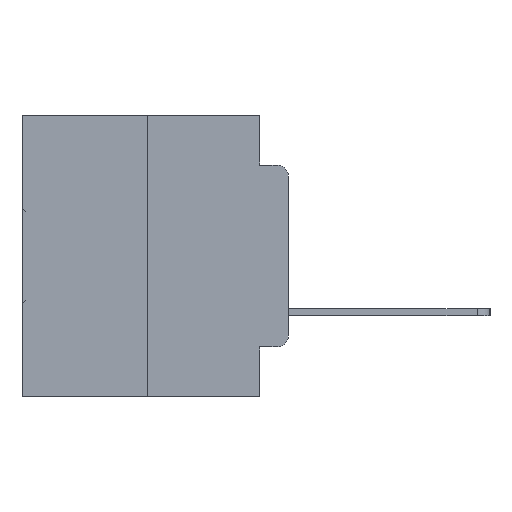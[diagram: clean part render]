
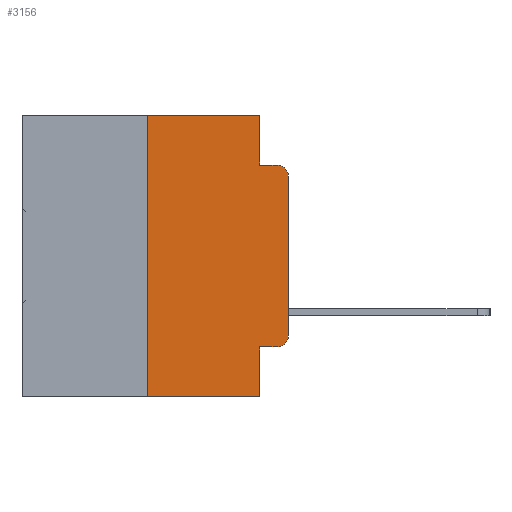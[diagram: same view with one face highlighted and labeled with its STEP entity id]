
A CAD part, left-side view. The second image highlights one B-rep face of the part: STEP entity #3156.
In plain terms, the highlighted planar face has unit normal (-1, 0, 0).
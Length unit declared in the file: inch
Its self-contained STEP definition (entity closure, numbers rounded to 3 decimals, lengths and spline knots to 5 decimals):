
#2211 = ORIENTED_EDGE ( 'NONE', *, *, #18443, .T. ) ;
#2408 = CARTESIAN_POINT ( 'NONE',  ( 0., 0.051, -0.4115 ) ) ;
#2585 = VECTOR ( 'NONE', #10073, 39.37008 ) ;
#2586 = VERTEX_POINT ( 'NONE', #30547 ) ;
#3156 = ADVANCED_FACE ( 'NONE', ( #18102 ), #22793, .F. ) ;
#3324 = DIRECTION ( 'NONE',  ( 0., -1., 0. ) ) ;
#3352 = CARTESIAN_POINT ( 'NONE',  ( 0., 0.25, -0.5 ) ) ;
#3470 = AXIS2_PLACEMENT_3D ( 'NONE', #5197, #27249, #27353 ) ;
#3489 = VERTEX_POINT ( 'NONE', #3352 ) ;
#3827 = CARTESIAN_POINT ( 'NONE',  ( 0., 0.02, -0.1085 ) ) ;
#4838 = CARTESIAN_POINT ( 'NONE',  ( 0., 0.02, -0.3915 ) ) ;
#5197 = CARTESIAN_POINT ( 'NONE',  ( 0., 0.473, 0. ) ) ;
#5593 = VECTOR ( 'NONE', #17565, 39.37008 ) ;
#6396 = DIRECTION ( 'NONE',  ( 0., 0., -1. ) ) ;
#6905 = CARTESIAN_POINT ( 'NONE',  ( 0., 0., -0.1085 ) ) ;
#7049 = VECTOR ( 'NONE', #3324, 39.37008 ) ;
#7392 = DIRECTION ( 'NONE',  ( 0., 0., -1. ) ) ;
#7925 = DIRECTION ( 'NONE',  ( 0., 0., -1. ) ) ;
#9530 = DIRECTION ( 'NONE',  ( 0., -1., 0. ) ) ;
#9537 = CARTESIAN_POINT ( 'NONE',  ( 0., 0.051, -0.4115 ) ) ;
#9700 = CARTESIAN_POINT ( 'NONE',  ( 0., 0.051, 0. ) ) ;
#10073 = DIRECTION ( 'NONE',  ( 0., 0., -1. ) ) ;
#10144 = ORIENTED_EDGE ( 'NONE', *, *, #25114, .F. ) ;
#10475 = LINE ( 'NONE', #30295, #16392 ) ;
#10679 = LINE ( 'NONE', #12119, #29667 ) ;
#12119 = CARTESIAN_POINT ( 'NONE',  ( 0., 0.473, 0. ) ) ;
#12227 = DIRECTION ( 'NONE',  ( 0., -1., 0. ) ) ;
#12269 = VERTEX_POINT ( 'NONE', #17184 ) ;
#12675 = DIRECTION ( 'NONE',  ( 0., 0., 1. ) ) ;
#12844 = VERTEX_POINT ( 'NONE', #9537 ) ;
#13385 = EDGE_CURVE ( 'NONE', #24748, #22468, #28639, .T. ) ;
#13548 = LINE ( 'NONE', #23791, #26031 ) ;
#14113 = ORIENTED_EDGE ( 'NONE', *, *, #21798, .F. ) ;
#14485 = ORIENTED_EDGE ( 'NONE', *, *, #31569, .T. ) ;
#14587 = LINE ( 'NONE', #23485, #7049 ) ;
#15309 = LINE ( 'NONE', #27521, #2585 ) ;
#15716 = ORIENTED_EDGE ( 'NONE', *, *, #13385, .T. ) ;
#15809 = VERTEX_POINT ( 'NONE', #9700 ) ;
#16392 = VECTOR ( 'NONE', #7925, 39.37008 ) ;
#17184 = CARTESIAN_POINT ( 'NONE',  ( 0., 0.051, -0.0885 ) ) ;
#17565 = DIRECTION ( 'NONE',  ( 0., -1., 0. ) ) ;
#18102 = FACE_OUTER_BOUND ( 'NONE', #30571, .T. ) ;
#18443 = EDGE_CURVE ( 'NONE', #12844, #24748, #31278, .T. ) ;
#18604 = VECTOR ( 'NONE', #12675, 39.37008 ) ;
#18692 = CARTESIAN_POINT ( 'NONE',  ( 0., 0.02, -0.4115 ) ) ;
#20120 = EDGE_CURVE ( 'NONE', #12844, #2586, #10475, .T. ) ;
#20365 = VERTEX_POINT ( 'NONE', #28921 ) ;
#20530 = LINE ( 'NONE', #24535, #21310 ) ;
#20780 = ORIENTED_EDGE ( 'NONE', *, *, #23865, .T. ) ;
#21310 = VECTOR ( 'NONE', #9530, 39.37008 ) ;
#21491 = DIRECTION ( 'NONE',  ( -1., 0., 0. ) ) ;
#21798 = EDGE_CURVE ( 'NONE', #3489, #32267, #25226, .T. ) ;
#21809 = CARTESIAN_POINT ( 'NONE',  ( 0., 0.25, 0. ) ) ;
#22468 = VERTEX_POINT ( 'NONE', #27749 ) ;
#22487 = DIRECTION ( 'NONE',  ( -1., 0., 0. ) ) ;
#22728 = ORIENTED_EDGE ( 'NONE', *, *, #26734, .F. ) ;
#22758 = CIRCLE ( 'NONE', #29147, 0.02 ) ;
#22793 = PLANE ( 'NONE',  #3470 ) ;
#23485 = CARTESIAN_POINT ( 'NONE',  ( 0., 0.473, -0.5 ) ) ;
#23531 = EDGE_CURVE ( 'NONE', #32267, #15809, #10679, .T. ) ;
#23791 = CARTESIAN_POINT ( 'NONE',  ( 0., 0., 0. ) ) ;
#23865 = EDGE_CURVE ( 'NONE', #3489, #2586, #14587, .T. ) ;
#24535 = CARTESIAN_POINT ( 'NONE',  ( 0., 0.051, -0.0885 ) ) ;
#24748 = VERTEX_POINT ( 'NONE', #18692 ) ;
#24809 = AXIS2_PLACEMENT_3D ( 'NONE', #4838, #22487, #7392 ) ;
#25039 = ORIENTED_EDGE ( 'NONE', *, *, #23531, .F. ) ;
#25114 = EDGE_CURVE ( 'NONE', #15809, #12269, #15309, .T. ) ;
#25226 = LINE ( 'NONE', #29984, #18604 ) ;
#26031 = VECTOR ( 'NONE', #28694, 39.37008 ) ;
#26092 = VERTEX_POINT ( 'NONE', #6905 ) ;
#26734 = EDGE_CURVE ( 'NONE', #12269, #20365, #20530, .T. ) ;
#27249 = DIRECTION ( 'NONE',  ( 1., 0., 0. ) ) ;
#27353 = DIRECTION ( 'NONE',  ( 0., 0., -1. ) ) ;
#27521 = CARTESIAN_POINT ( 'NONE',  ( 0., 0.051, 0. ) ) ;
#27689 = ORIENTED_EDGE ( 'NONE', *, *, #28355, .T. ) ;
#27749 = CARTESIAN_POINT ( 'NONE',  ( 0., 0., -0.3915 ) ) ;
#28084 = ORIENTED_EDGE ( 'NONE', *, *, #20120, .F. ) ;
#28355 = EDGE_CURVE ( 'NONE', #26092, #20365, #22758, .T. ) ;
#28639 = CIRCLE ( 'NONE', #24809, 0.02 ) ;
#28694 = DIRECTION ( 'NONE',  ( 0., 0., 1. ) ) ;
#28921 = CARTESIAN_POINT ( 'NONE',  ( 0., 0.02, -0.0885 ) ) ;
#29147 = AXIS2_PLACEMENT_3D ( 'NONE', #3827, #21491, #6396 ) ;
#29667 = VECTOR ( 'NONE', #12227, 39.37008 ) ;
#29984 = CARTESIAN_POINT ( 'NONE',  ( 0., 0.25, 0. ) ) ;
#30295 = CARTESIAN_POINT ( 'NONE',  ( 0., 0.051, 0. ) ) ;
#30547 = CARTESIAN_POINT ( 'NONE',  ( 0., 0.051, -0.5 ) ) ;
#30571 = EDGE_LOOP ( 'NONE', ( #14485, #27689, #22728, #10144, #25039, #14113, #20780, #28084, #2211, #15716 ) ) ;
#31278 = LINE ( 'NONE', #2408, #5593 ) ;
#31569 = EDGE_CURVE ( 'NONE', #22468, #26092, #13548, .T. ) ;
#32267 = VERTEX_POINT ( 'NONE', #21809 ) ;
